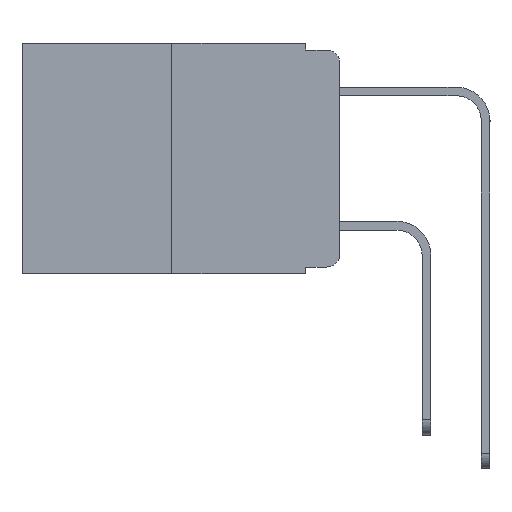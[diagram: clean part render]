
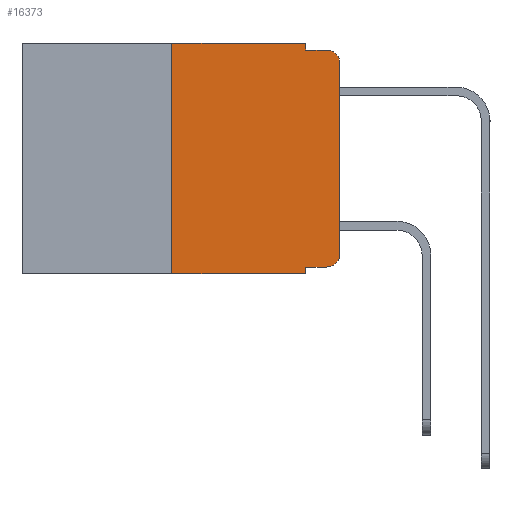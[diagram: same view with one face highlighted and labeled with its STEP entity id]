
A CAD part, left-side view. The second image highlights one B-rep face of the part: STEP entity #16373.
In plain terms, the highlighted planar face has unit normal (-1, 0, 0).
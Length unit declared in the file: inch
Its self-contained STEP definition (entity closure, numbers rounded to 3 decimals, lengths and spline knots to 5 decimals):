
#748 = CARTESIAN_POINT ( 'NONE',  ( 0., 0.051, -0.343 ) ) ;
#842 = VERTEX_POINT ( 'NONE', #10907 ) ;
#1000 = EDGE_CURVE ( 'NONE', #15670, #24227, #15779, .T. ) ;
#1175 = DIRECTION ( 'NONE',  ( 0., -1., 0. ) ) ;
#1201 = FACE_OUTER_BOUND ( 'NONE', #14084, .T. ) ;
#1423 = VERTEX_POINT ( 'NONE', #748 ) ;
#1638 = CARTESIAN_POINT ( 'NONE',  ( 0., 0., -0.03 ) ) ;
#1777 = AXIS2_PLACEMENT_3D ( 'NONE', #13991, #2046, #15992 ) ;
#2013 = ORIENTED_EDGE ( 'NONE', *, *, #24195, .F. ) ;
#2046 = DIRECTION ( 'NONE',  ( 1., 0., 0. ) ) ;
#2987 = CARTESIAN_POINT ( 'NONE',  ( 0., 0., 0. ) ) ;
#3019 = DIRECTION ( 'NONE',  ( 0., 0., 1. ) ) ;
#3715 = EDGE_CURVE ( 'NONE', #25665, #15670, #5672, .T. ) ;
#3788 = DIRECTION ( 'NONE',  ( 0., -1., 0. ) ) ;
#4221 = LINE ( 'NONE', #13132, #14811 ) ;
#4340 = LINE ( 'NONE', #17502, #24859 ) ;
#4506 = CARTESIAN_POINT ( 'NONE',  ( 0., 0.473, -0.343 ) ) ;
#4703 = LINE ( 'NONE', #21153, #9371 ) ;
#4814 = ORIENTED_EDGE ( 'NONE', *, *, #3715, .T. ) ;
#5123 = VECTOR ( 'NONE', #22323, 39.37008 ) ;
#5298 = VECTOR ( 'NONE', #3788, 39.37008 ) ;
#5455 = ORIENTED_EDGE ( 'NONE', *, *, #1000, .T. ) ;
#5489 = CIRCLE ( 'NONE', #14367, 0.02 ) ;
#5558 = EDGE_CURVE ( 'NONE', #20464, #24310, #20576, .T. ) ;
#5672 = LINE ( 'NONE', #2987, #21563 ) ;
#5786 = EDGE_CURVE ( 'NONE', #16562, #17941, #15718, .T. ) ;
#6758 = PLANE ( 'NONE',  #1777 ) ;
#6809 = CARTESIAN_POINT ( 'NONE',  ( 0., 0.25, -0.343 ) ) ;
#7237 = CARTESIAN_POINT ( 'NONE',  ( 0., 0.02, -0.313 ) ) ;
#7315 = VECTOR ( 'NONE', #20469, 39.37008 ) ;
#8543 = LINE ( 'NONE', #4506, #7315 ) ;
#8569 = ORIENTED_EDGE ( 'NONE', *, *, #16240, .F. ) ;
#9215 = DIRECTION ( 'NONE',  ( 0., 0., -1. ) ) ;
#9371 = VECTOR ( 'NONE', #25089, 39.37008 ) ;
#9539 = CARTESIAN_POINT ( 'NONE',  ( 0., 0.02, -0.333 ) ) ;
#9809 = CARTESIAN_POINT ( 'NONE',  ( 0., 0., -0.313 ) ) ;
#10123 = ORIENTED_EDGE ( 'NONE', *, *, #17582, .F. ) ;
#10367 = CARTESIAN_POINT ( 'NONE',  ( 0., 0.473, 0. ) ) ;
#10796 = DIRECTION ( 'NONE',  ( 0., 0., -1. ) ) ;
#10817 = DIRECTION ( 'NONE',  ( -1., 0., 0. ) ) ;
#10823 = CARTESIAN_POINT ( 'NONE',  ( 0., 0.02, -0.03 ) ) ;
#10907 = CARTESIAN_POINT ( 'NONE',  ( 0., 0.051, -0.01 ) ) ;
#11361 = EDGE_CURVE ( 'NONE', #24310, #25665, #5489, .T. ) ;
#12293 = DIRECTION ( 'NONE',  ( 0., 0., 1. ) ) ;
#12572 = CARTESIAN_POINT ( 'NONE',  ( 0., 0.25, 0. ) ) ;
#12604 = ORIENTED_EDGE ( 'NONE', *, *, #20259, .F. ) ;
#13011 = VECTOR ( 'NONE', #12293, 39.37008 ) ;
#13132 = CARTESIAN_POINT ( 'NONE',  ( 0., 0.051, -0.01 ) ) ;
#13430 = CARTESIAN_POINT ( 'NONE',  ( 0., 0.051, 0. ) ) ;
#13991 = CARTESIAN_POINT ( 'NONE',  ( 0., 0.473, 0. ) ) ;
#14084 = EDGE_LOOP ( 'NONE', ( #4814, #5455, #2013, #12604, #14810, #10123, #23236, #8569, #19843, #25042 ) ) ;
#14367 = AXIS2_PLACEMENT_3D ( 'NONE', #7237, #21172, #9215 ) ;
#14810 = ORIENTED_EDGE ( 'NONE', *, *, #5786, .F. ) ;
#14811 = VECTOR ( 'NONE', #1175, 39.37008 ) ;
#15670 = VERTEX_POINT ( 'NONE', #1638 ) ;
#15711 = CARTESIAN_POINT ( 'NONE',  ( 0., 0.051, -0.333 ) ) ;
#15718 = LINE ( 'NONE', #10367, #5123 ) ;
#15779 = CIRCLE ( 'NONE', #23586, 0.02 ) ;
#15992 = DIRECTION ( 'NONE',  ( 0., 0., -1. ) ) ;
#16240 = EDGE_CURVE ( 'NONE', #20464, #1423, #4340, .T. ) ;
#16373 = ADVANCED_FACE ( 'NONE', ( #1201 ), #6758, .F. ) ;
#16562 = VERTEX_POINT ( 'NONE', #12572 ) ;
#17288 = CARTESIAN_POINT ( 'NONE',  ( 0., 0.051, -0.333 ) ) ;
#17502 = CARTESIAN_POINT ( 'NONE',  ( 0., 0.051, 0. ) ) ;
#17582 = EDGE_CURVE ( 'NONE', #23450, #16562, #23597, .T. ) ;
#17941 = VERTEX_POINT ( 'NONE', #13430 ) ;
#18255 = CARTESIAN_POINT ( 'NONE',  ( 0., 0.25, 0. ) ) ;
#18269 = EDGE_CURVE ( 'NONE', #23450, #1423, #8543, .T. ) ;
#19516 = DIRECTION ( 'NONE',  ( 0., 0., -1. ) ) ;
#19843 = ORIENTED_EDGE ( 'NONE', *, *, #5558, .T. ) ;
#20259 = EDGE_CURVE ( 'NONE', #17941, #842, #4703, .T. ) ;
#20464 = VERTEX_POINT ( 'NONE', #17288 ) ;
#20469 = DIRECTION ( 'NONE',  ( 0., -1., 0. ) ) ;
#20576 = LINE ( 'NONE', #15711, #5298 ) ;
#21153 = CARTESIAN_POINT ( 'NONE',  ( 0., 0.051, 0. ) ) ;
#21172 = DIRECTION ( 'NONE',  ( -1., 0., 0. ) ) ;
#21563 = VECTOR ( 'NONE', #3019, 39.37008 ) ;
#22323 = DIRECTION ( 'NONE',  ( 0., -1., 0. ) ) ;
#23236 = ORIENTED_EDGE ( 'NONE', *, *, #18269, .T. ) ;
#23450 = VERTEX_POINT ( 'NONE', #6809 ) ;
#23586 = AXIS2_PLACEMENT_3D ( 'NONE', #10823, #10817, #10796 ) ;
#23597 = LINE ( 'NONE', #18255, #13011 ) ;
#24195 = EDGE_CURVE ( 'NONE', #842, #24227, #4221, .T. ) ;
#24227 = VERTEX_POINT ( 'NONE', #25084 ) ;
#24310 = VERTEX_POINT ( 'NONE', #9539 ) ;
#24859 = VECTOR ( 'NONE', #19516, 39.37008 ) ;
#25042 = ORIENTED_EDGE ( 'NONE', *, *, #11361, .T. ) ;
#25084 = CARTESIAN_POINT ( 'NONE',  ( 0., 0.02, -0.01 ) ) ;
#25089 = DIRECTION ( 'NONE',  ( 0., 0., -1. ) ) ;
#25665 = VERTEX_POINT ( 'NONE', #9809 ) ;
